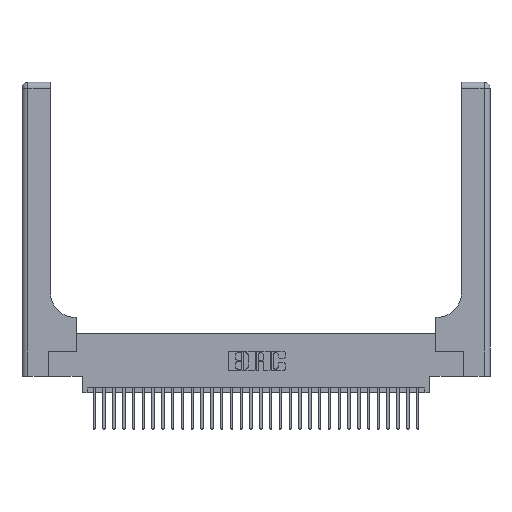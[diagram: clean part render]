
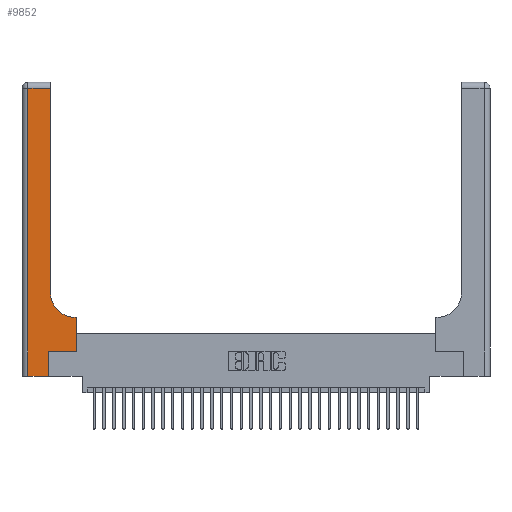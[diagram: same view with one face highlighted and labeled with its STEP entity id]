
A CAD part, top view. The second image highlights one B-rep face of the part: STEP entity #9852.
In plain terms, the highlighted planar face has unit normal (0, 0, 1).
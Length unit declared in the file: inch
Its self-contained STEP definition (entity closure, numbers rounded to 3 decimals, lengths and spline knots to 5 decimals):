
#541 = VERTEX_POINT ( 'NONE', #2092 ) ;
#764 = CARTESIAN_POINT ( 'NONE',  ( 0.5415, 0.6, 0.37 ) ) ;
#966 = LINE ( 'NONE', #24439, #7832 ) ;
#1263 = EDGE_CURVE ( 'NONE', #19803, #541, #28974, .T. ) ;
#1729 = EDGE_LOOP ( 'NONE', ( #23313, #11656, #23034, #26800, #27840, #21658, #24348, #32515, #2308 ) ) ;
#1877 = CARTESIAN_POINT ( 'NONE',  ( 0.269, 0.25, 0.37 ) ) ;
#2092 = CARTESIAN_POINT ( 'NONE',  ( 0.06, 2.94, 0.37 ) ) ;
#2176 = DIRECTION ( 'NONE',  ( 0., 1., 0. ) ) ;
#2308 = ORIENTED_EDGE ( 'NONE', *, *, #12102, .T. ) ;
#2379 = CARTESIAN_POINT ( 'NONE',  ( 0.2915, 0.85, 0.37 ) ) ;
#2552 = VECTOR ( 'NONE', #2176, 39.37008 ) ;
#2923 = CARTESIAN_POINT ( 'NONE',  ( 0., 3., 0.37 ) ) ;
#3330 = DIRECTION ( 'NONE',  ( 0., 1., 0. ) ) ;
#3413 = VECTOR ( 'NONE', #3330, 39.37008 ) ;
#4113 = LINE ( 'NONE', #8617, #17674 ) ;
#5505 = DIRECTION ( 'NONE',  ( -1., 0., 0. ) ) ;
#7534 = VERTEX_POINT ( 'NONE', #18611 ) ;
#7832 = VECTOR ( 'NONE', #11739, 39.37008 ) ;
#8594 = EDGE_CURVE ( 'NONE', #15067, #7534, #29746, .T. ) ;
#8617 = CARTESIAN_POINT ( 'NONE',  ( 0., 0., 0.37 ) ) ;
#8660 = CARTESIAN_POINT ( 'NONE',  ( 0.5585, 0.25, 0.37 ) ) ;
#9464 = VECTOR ( 'NONE', #25032, 39.37008 ) ;
#9852 = ADVANCED_FACE ( 'NONE', ( #23590 ), #15664, .F. ) ;
#11052 = CARTESIAN_POINT ( 'NONE',  ( 0.5585, 0.25, 0.37 ) ) ;
#11656 = ORIENTED_EDGE ( 'NONE', *, *, #1263, .T. ) ;
#11739 = DIRECTION ( 'NONE',  ( -1., 0., 0. ) ) ;
#12078 = CARTESIAN_POINT ( 'NONE',  ( 0.269, 0.25, 0.37 ) ) ;
#12102 = EDGE_CURVE ( 'NONE', #19345, #20238, #29816, .T. ) ;
#12224 = CARTESIAN_POINT ( 'NONE',  ( 0., 2.94, 0.37 ) ) ;
#12429 = LINE ( 'NONE', #23115, #18394 ) ;
#12483 = CARTESIAN_POINT ( 'NONE',  ( 0.5415, 0.85, 0.37 ) ) ;
#13143 = EDGE_CURVE ( 'NONE', #7534, #19345, #966, .T. ) ;
#15037 = DIRECTION ( 'NONE',  ( 1., 0., 0. ) ) ;
#15067 = VERTEX_POINT ( 'NONE', #8660 ) ;
#15617 = EDGE_CURVE ( 'NONE', #26600, #28937, #4113, .T. ) ;
#15664 = PLANE ( 'NONE',  #29910 ) ;
#16101 = DIRECTION ( 'NONE',  ( 1., 0., 0. ) ) ;
#16939 = CARTESIAN_POINT ( 'NONE',  ( 0.06, 3., 0.37 ) ) ;
#17674 = VECTOR ( 'NONE', #16101, 39.37008 ) ;
#17761 = VERTEX_POINT ( 'NONE', #12078 ) ;
#18394 = VECTOR ( 'NONE', #25694, 39.37008 ) ;
#18611 = CARTESIAN_POINT ( 'NONE',  ( 0.5585, 0.6, 0.37 ) ) ;
#19345 = VERTEX_POINT ( 'NONE', #764 ) ;
#19803 = VERTEX_POINT ( 'NONE', #22868 ) ;
#19814 = CARTESIAN_POINT ( 'NONE',  ( 0.269, 0., 0.37 ) ) ;
#20238 = VERTEX_POINT ( 'NONE', #2379 ) ;
#20750 = DIRECTION ( 'NONE',  ( 0., 0., -1. ) ) ;
#20946 = VECTOR ( 'NONE', #22285, 39.37008 ) ;
#21658 = ORIENTED_EDGE ( 'NONE', *, *, #30127, .T. ) ;
#21765 = LINE ( 'NONE', #1877, #20946 ) ;
#22054 = EDGE_CURVE ( 'NONE', #20238, #19803, #12429, .T. ) ;
#22285 = DIRECTION ( 'NONE',  ( 1., 0., 0. ) ) ;
#22578 = CARTESIAN_POINT ( 'NONE',  ( 0.269, 0., 0.37 ) ) ;
#22868 = CARTESIAN_POINT ( 'NONE',  ( 0.2915, 2.94, 0.37 ) ) ;
#23034 = ORIENTED_EDGE ( 'NONE', *, *, #28882, .T. ) ;
#23115 = CARTESIAN_POINT ( 'NONE',  ( 0.2915, 3., 0.37 ) ) ;
#23313 = ORIENTED_EDGE ( 'NONE', *, *, #22054, .T. ) ;
#23590 = FACE_OUTER_BOUND ( 'NONE', #1729, .T. ) ;
#24348 = ORIENTED_EDGE ( 'NONE', *, *, #8594, .T. ) ;
#24439 = CARTESIAN_POINT ( 'NONE',  ( 0.2915, 0.6, 0.37 ) ) ;
#25032 = DIRECTION ( 'NONE',  ( -1., 0., 0. ) ) ;
#25694 = DIRECTION ( 'NONE',  ( 0., 1., 0. ) ) ;
#26102 = AXIS2_PLACEMENT_3D ( 'NONE', #12483, #30285, #15037 ) ;
#26600 = VERTEX_POINT ( 'NONE', #30569 ) ;
#26800 = ORIENTED_EDGE ( 'NONE', *, *, #15617, .T. ) ;
#27840 = ORIENTED_EDGE ( 'NONE', *, *, #30789, .T. ) ;
#28882 = EDGE_CURVE ( 'NONE', #541, #26600, #30619, .T. ) ;
#28888 = LINE ( 'NONE', #22578, #2552 ) ;
#28937 = VERTEX_POINT ( 'NONE', #19814 ) ;
#28974 = LINE ( 'NONE', #12224, #9464 ) ;
#29746 = LINE ( 'NONE', #11052, #3413 ) ;
#29816 = CIRCLE ( 'NONE', #26102, 0.25 ) ;
#29827 = VECTOR ( 'NONE', #32279, 39.37008 ) ;
#29910 = AXIS2_PLACEMENT_3D ( 'NONE', #2923, #20750, #5505 ) ;
#30127 = EDGE_CURVE ( 'NONE', #17761, #15067, #21765, .T. ) ;
#30285 = DIRECTION ( 'NONE',  ( 0., 0., -1. ) ) ;
#30569 = CARTESIAN_POINT ( 'NONE',  ( 0.06, 0., 0.37 ) ) ;
#30619 = LINE ( 'NONE', #16939, #29827 ) ;
#30789 = EDGE_CURVE ( 'NONE', #28937, #17761, #28888, .T. ) ;
#32279 = DIRECTION ( 'NONE',  ( 0., -1., 0. ) ) ;
#32515 = ORIENTED_EDGE ( 'NONE', *, *, #13143, .T. ) ;
